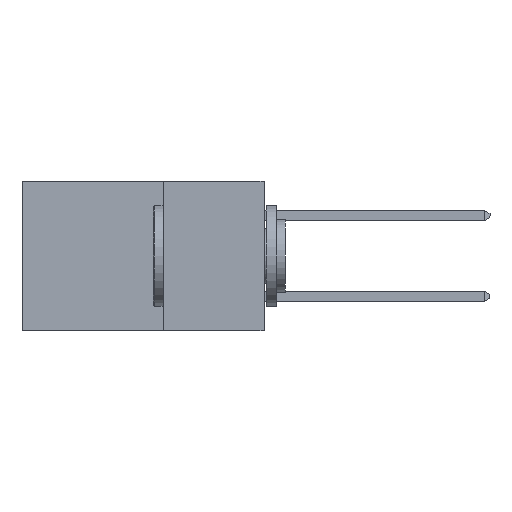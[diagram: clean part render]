
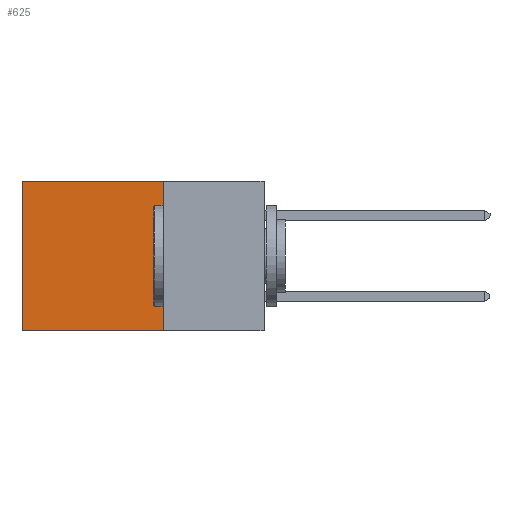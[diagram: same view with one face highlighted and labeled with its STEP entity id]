
A CAD part, left-side view. The second image highlights one B-rep face of the part: STEP entity #625.
In plain terms, the highlighted planar face has unit normal (-1, 0, 0).
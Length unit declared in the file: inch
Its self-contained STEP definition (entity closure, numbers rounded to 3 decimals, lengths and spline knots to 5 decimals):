
#240 = ORIENTED_EDGE ( 'NONE', *, *, #971, .T. ) ;
#311 = ORIENTED_EDGE ( 'NONE', *, *, #5439, .F. ) ;
#625 = ADVANCED_FACE ( 'NONE', ( #11178 ), #14156, .F. ) ;
#971 = EDGE_CURVE ( 'NONE', #13371, #6625, #2992, .T. ) ;
#1071 = EDGE_CURVE ( 'NONE', #13371, #7225, #10829, .T. ) ;
#1090 = ORIENTED_EDGE ( 'NONE', *, *, #9397, .T. ) ;
#1420 = CARTESIAN_POINT ( 'NONE',  ( 0.298, 0.25, 0. ) ) ;
#1606 = VECTOR ( 'NONE', #14442, 39.37008 ) ;
#1707 = CARTESIAN_POINT ( 'NONE',  ( 0.298, 0.6, 0. ) ) ;
#1877 = DIRECTION ( 'NONE',  ( 0., 0., -1. ) ) ;
#2072 = CARTESIAN_POINT ( 'NONE',  ( 0.298, 0.6, -0.37 ) ) ;
#2518 = CARTESIAN_POINT ( 'NONE',  ( 0.298, 0.6, 0. ) ) ;
#2542 = CARTESIAN_POINT ( 'NONE',  ( 0.298, 0.25, -0.37 ) ) ;
#2698 = VECTOR ( 'NONE', #5568, 39.37008 ) ;
#2992 = LINE ( 'NONE', #14132, #7806 ) ;
#3257 = LINE ( 'NONE', #1707, #12152 ) ;
#5439 = EDGE_CURVE ( 'NONE', #7225, #11403, #14241, .T. ) ;
#5568 = DIRECTION ( 'NONE',  ( 0., 1., 0. ) ) ;
#5598 = ORIENTED_EDGE ( 'NONE', *, *, #1071, .F. ) ;
#6625 = VERTEX_POINT ( 'NONE', #2518 ) ;
#7225 = VERTEX_POINT ( 'NONE', #11182 ) ;
#7416 = DIRECTION ( 'NONE',  ( 0., 1., 0. ) ) ;
#7806 = VECTOR ( 'NONE', #7416, 39.37008 ) ;
#9397 = EDGE_CURVE ( 'NONE', #6625, #11403, #3257, .T. ) ;
#10829 = LINE ( 'NONE', #14047, #1606 ) ;
#11178 = FACE_OUTER_BOUND ( 'NONE', #11581, .T. ) ;
#11182 = CARTESIAN_POINT ( 'NONE',  ( 0.298, 0.25, -0.37 ) ) ;
#11403 = VERTEX_POINT ( 'NONE', #2072 ) ;
#11581 = EDGE_LOOP ( 'NONE', ( #1090, #311, #5598, #240 ) ) ;
#12152 = VECTOR ( 'NONE', #1877, 39.37008 ) ;
#13081 = CARTESIAN_POINT ( 'NONE',  ( 0.298, 0.25, 0. ) ) ;
#13111 = DIRECTION ( 'NONE',  ( 1., 0., 0. ) ) ;
#13171 = DIRECTION ( 'NONE',  ( 0., 0., -1. ) ) ;
#13371 = VERTEX_POINT ( 'NONE', #1420 ) ;
#13672 = AXIS2_PLACEMENT_3D ( 'NONE', #13081, #13111, #13171 ) ;
#14047 = CARTESIAN_POINT ( 'NONE',  ( 0.298, 0.25, 0. ) ) ;
#14132 = CARTESIAN_POINT ( 'NONE',  ( 0.298, 0.25, 0. ) ) ;
#14156 = PLANE ( 'NONE',  #13672 ) ;
#14241 = LINE ( 'NONE', #2542, #2698 ) ;
#14442 = DIRECTION ( 'NONE',  ( 0., 0., -1. ) ) ;
